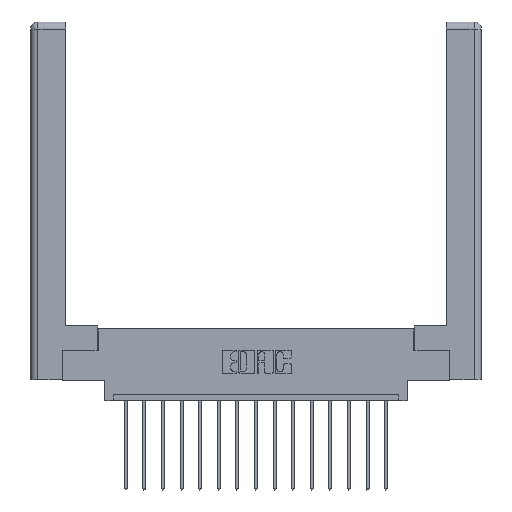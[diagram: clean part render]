
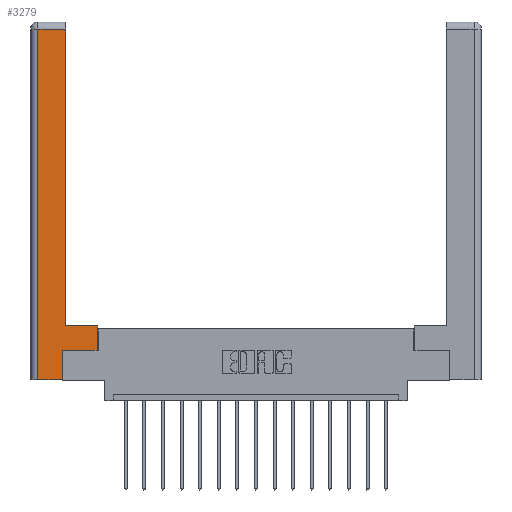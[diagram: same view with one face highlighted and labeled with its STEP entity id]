
A CAD part, top view. The second image highlights one B-rep face of the part: STEP entity #3279.
In plain terms, the highlighted planar face has unit normal (0, 0, 1).
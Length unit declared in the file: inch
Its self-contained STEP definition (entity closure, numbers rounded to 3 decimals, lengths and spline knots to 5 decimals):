
#153 = DIRECTION ( 'NONE',  ( 0., -1., 0. ) ) ;
#306 = VECTOR ( 'NONE', #5238, 39.37008 ) ;
#402 = CARTESIAN_POINT ( 'NONE',  ( 0.295, 2.94, 0. ) ) ;
#703 = CARTESIAN_POINT ( 'NONE',  ( 0.265, 0.245, 0. ) ) ;
#1096 = EDGE_CURVE ( 'NONE', #14688, #16630, #1860, .T. ) ;
#1177 = VECTOR ( 'NONE', #9669, 39.37008 ) ;
#1245 = VECTOR ( 'NONE', #4723, 39.37008 ) ;
#1368 = VECTOR ( 'NONE', #153, 39.37008 ) ;
#1525 = VERTEX_POINT ( 'NONE', #12832 ) ;
#1860 = LINE ( 'NONE', #14113, #1245 ) ;
#1901 = EDGE_CURVE ( 'NONE', #3728, #8841, #11927, .T. ) ;
#2668 = ORIENTED_EDGE ( 'NONE', *, *, #15646, .T. ) ;
#2733 = PLANE ( 'NONE',  #11867 ) ;
#2816 = FACE_OUTER_BOUND ( 'NONE', #13268, .T. ) ;
#2902 = CARTESIAN_POINT ( 'NONE',  ( 0.0615, 0., 0. ) ) ;
#3279 = ADVANCED_FACE ( 'NONE', ( #2816 ), #2733, .F. ) ;
#3728 = VERTEX_POINT ( 'NONE', #10483 ) ;
#3835 = LINE ( 'NONE', #7887, #6092 ) ;
#4514 = VERTEX_POINT ( 'NONE', #402 ) ;
#4723 = DIRECTION ( 'NONE',  ( 1., 0., 0. ) ) ;
#4757 = CARTESIAN_POINT ( 'NONE',  ( 0.0615, 2.94, 0. ) ) ;
#4922 = CARTESIAN_POINT ( 'NONE',  ( 0.265, 0., 0. ) ) ;
#5138 = CARTESIAN_POINT ( 'NONE',  ( 0.295, 3., 0. ) ) ;
#5150 = LINE ( 'NONE', #5138, #17400 ) ;
#5238 = DIRECTION ( 'NONE',  ( 0., 1., 0. ) ) ;
#5354 = DIRECTION ( 'NONE',  ( -1., 0., 0. ) ) ;
#5397 = DIRECTION ( 'NONE',  ( -1., 0., 0. ) ) ;
#6092 = VECTOR ( 'NONE', #10505, 39.37008 ) ;
#6316 = CARTESIAN_POINT ( 'NONE',  ( 0.0615, 0., 0. ) ) ;
#7384 = LINE ( 'NONE', #703, #15865 ) ;
#7887 = CARTESIAN_POINT ( 'NONE',  ( 0.0615, 2.94, 0. ) ) ;
#8429 = CARTESIAN_POINT ( 'NONE',  ( 0.265, 0.245, 0. ) ) ;
#8841 = VERTEX_POINT ( 'NONE', #11317 ) ;
#9533 = CARTESIAN_POINT ( 'NONE',  ( 0.295, 0.45, 0. ) ) ;
#9669 = DIRECTION ( 'NONE',  ( 1., 0., 0. ) ) ;
#10310 = EDGE_CURVE ( 'NONE', #1525, #3728, #15258, .T. ) ;
#10483 = CARTESIAN_POINT ( 'NONE',  ( 0.565, 0.45, 0. ) ) ;
#10505 = DIRECTION ( 'NONE',  ( -1., 0., 0. ) ) ;
#10717 = VERTEX_POINT ( 'NONE', #4757 ) ;
#11317 = CARTESIAN_POINT ( 'NONE',  ( 0.295, 0.45, 0. ) ) ;
#11439 = ORIENTED_EDGE ( 'NONE', *, *, #10310, .T. ) ;
#11589 = EDGE_CURVE ( 'NONE', #4514, #10717, #3835, .T. ) ;
#11867 = AXIS2_PLACEMENT_3D ( 'NONE', #12260, #14913, #5397 ) ;
#11927 = LINE ( 'NONE', #9533, #13601 ) ;
#12260 = CARTESIAN_POINT ( 'NONE',  ( 0., 0., 0. ) ) ;
#12832 = CARTESIAN_POINT ( 'NONE',  ( 0.565, 0.245, 0. ) ) ;
#12940 = LINE ( 'NONE', #2902, #1368 ) ;
#13268 = EDGE_LOOP ( 'NONE', ( #15788, #15395, #17141, #15366, #15336, #2668, #11439, #13975 ) ) ;
#13601 = VECTOR ( 'NONE', #5354, 39.37008 ) ;
#13975 = ORIENTED_EDGE ( 'NONE', *, *, #1901, .T. ) ;
#14046 = VERTEX_POINT ( 'NONE', #8429 ) ;
#14113 = CARTESIAN_POINT ( 'NONE',  ( 0.265, 0., 0. ) ) ;
#14224 = DIRECTION ( 'NONE',  ( 0., 1., 0. ) ) ;
#14688 = VERTEX_POINT ( 'NONE', #6316 ) ;
#14712 = DIRECTION ( 'NONE',  ( 0., 1., 0. ) ) ;
#14913 = DIRECTION ( 'NONE',  ( 0., 0., -1. ) ) ;
#15258 = LINE ( 'NONE', #17166, #306 ) ;
#15336 = ORIENTED_EDGE ( 'NONE', *, *, #16950, .T. ) ;
#15366 = ORIENTED_EDGE ( 'NONE', *, *, #1096, .T. ) ;
#15395 = ORIENTED_EDGE ( 'NONE', *, *, #11589, .T. ) ;
#15456 = EDGE_CURVE ( 'NONE', #8841, #4514, #5150, .T. ) ;
#15488 = LINE ( 'NONE', #16393, #1177 ) ;
#15646 = EDGE_CURVE ( 'NONE', #14046, #1525, #15488, .T. ) ;
#15788 = ORIENTED_EDGE ( 'NONE', *, *, #15456, .T. ) ;
#15865 = VECTOR ( 'NONE', #14224, 39.37008 ) ;
#16224 = EDGE_CURVE ( 'NONE', #10717, #14688, #12940, .T. ) ;
#16393 = CARTESIAN_POINT ( 'NONE',  ( 0.565, 0.245, 0. ) ) ;
#16630 = VERTEX_POINT ( 'NONE', #4922 ) ;
#16950 = EDGE_CURVE ( 'NONE', #16630, #14046, #7384, .T. ) ;
#17141 = ORIENTED_EDGE ( 'NONE', *, *, #16224, .T. ) ;
#17166 = CARTESIAN_POINT ( 'NONE',  ( 0.565, 0.45, 0. ) ) ;
#17400 = VECTOR ( 'NONE', #14712, 39.37008 ) ;
